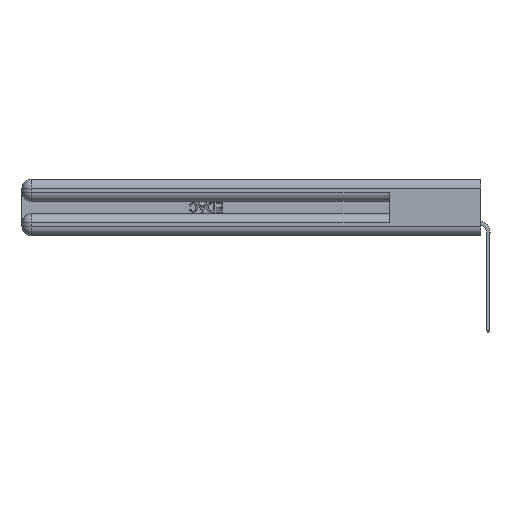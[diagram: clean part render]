
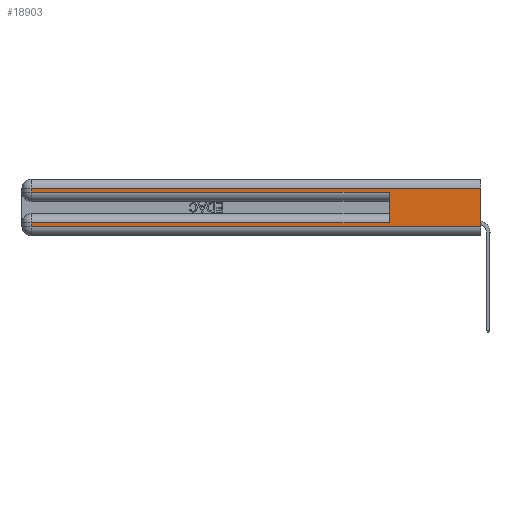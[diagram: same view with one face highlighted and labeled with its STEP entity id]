
A CAD part, left-side view. The second image highlights one B-rep face of the part: STEP entity #18903.
In plain terms, the highlighted planar face has unit normal (-1, 0, 0).
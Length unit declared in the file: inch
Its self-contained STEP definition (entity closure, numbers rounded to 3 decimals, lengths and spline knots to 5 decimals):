
#931 = ORIENTED_EDGE ( 'NONE', *, *, #13515, .T. ) ;
#1380 = EDGE_CURVE ( 'NONE', #7240, #13594, #26486, .T. ) ;
#1439 = VECTOR ( 'NONE', #4902, 39.37008 ) ;
#1714 = CARTESIAN_POINT ( 'NONE',  ( 0., 2.94, 0.31 ) ) ;
#1942 = VECTOR ( 'NONE', #2639, 39.37008 ) ;
#2200 = DIRECTION ( 'NONE',  ( 0., 0., -1. ) ) ;
#2639 = DIRECTION ( 'NONE',  ( 0., 0., 1. ) ) ;
#2645 = LINE ( 'NONE', #15497, #1439 ) ;
#2689 = VERTEX_POINT ( 'NONE', #3376 ) ;
#3376 = CARTESIAN_POINT ( 'NONE',  ( 0., 0., 0.31 ) ) ;
#4289 = CARTESIAN_POINT ( 'NONE',  ( 0., 0., 0.37 ) ) ;
#4371 = EDGE_CURVE ( 'NONE', #7240, #5179, #33213, .T. ) ;
#4902 = DIRECTION ( 'NONE',  ( 0., -1., 0. ) ) ;
#5179 = VERTEX_POINT ( 'NONE', #25873 ) ;
#5207 = EDGE_CURVE ( 'NONE', #2689, #12162, #29871, .T. ) ;
#6254 = CARTESIAN_POINT ( 'NONE',  ( 0., 0.6, 0.085 ) ) ;
#7240 = VERTEX_POINT ( 'NONE', #6254 ) ;
#7918 = LINE ( 'NONE', #9277, #29573 ) ;
#8537 = ORIENTED_EDGE ( 'NONE', *, *, #27252, .F. ) ;
#9277 = CARTESIAN_POINT ( 'NONE',  ( 0., 2.94, 0.37 ) ) ;
#9321 = CARTESIAN_POINT ( 'NONE',  ( 0., 0., 0.06 ) ) ;
#10846 = VERTEX_POINT ( 'NONE', #32232 ) ;
#11100 = CARTESIAN_POINT ( 'NONE',  ( 0., 0.6, 0.285 ) ) ;
#11950 = VERTEX_POINT ( 'NONE', #21241 ) ;
#12162 = VERTEX_POINT ( 'NONE', #1714 ) ;
#12585 = FACE_OUTER_BOUND ( 'NONE', #28027, .T. ) ;
#12938 = CARTESIAN_POINT ( 'NONE',  ( 0., 0., 0.06 ) ) ;
#13391 = VECTOR ( 'NONE', #2200, 39.37008 ) ;
#13396 = DIRECTION ( 'NONE',  ( 0., 1., 0. ) ) ;
#13515 = EDGE_CURVE ( 'NONE', #12162, #11950, #13818, .T. ) ;
#13594 = VERTEX_POINT ( 'NONE', #11100 ) ;
#13818 = LINE ( 'NONE', #28677, #13391 ) ;
#14566 = PLANE ( 'NONE',  #22147 ) ;
#14887 = ORIENTED_EDGE ( 'NONE', *, *, #5207, .T. ) ;
#15438 = DIRECTION ( 'NONE',  ( 0., -1., 0. ) ) ;
#15471 = EDGE_CURVE ( 'NONE', #11950, #13594, #2645, .T. ) ;
#15497 = CARTESIAN_POINT ( 'NONE',  ( 0., 0., 0.285 ) ) ;
#15861 = ORIENTED_EDGE ( 'NONE', *, *, #32471, .T. ) ;
#17479 = DIRECTION ( 'NONE',  ( 0., 0., -1. ) ) ;
#17927 = DIRECTION ( 'NONE',  ( 0., 1., 0. ) ) ;
#18652 = CARTESIAN_POINT ( 'NONE',  ( 0., 0., 0.31 ) ) ;
#18903 = ADVANCED_FACE ( 'NONE', ( #12585 ), #14566, .F. ) ;
#19794 = ORIENTED_EDGE ( 'NONE', *, *, #15471, .T. ) ;
#20044 = DIRECTION ( 'NONE',  ( 1., 0., 0. ) ) ;
#20277 = VECTOR ( 'NONE', #24504, 39.37008 ) ;
#21241 = CARTESIAN_POINT ( 'NONE',  ( 0., 2.94, 0.285 ) ) ;
#21288 = VECTOR ( 'NONE', #13396, 39.37008 ) ;
#21293 = LINE ( 'NONE', #12938, #31121 ) ;
#22147 = AXIS2_PLACEMENT_3D ( 'NONE', #4289, #20044, #32945 ) ;
#22194 = CARTESIAN_POINT ( 'NONE',  ( 0., 0., 0.085 ) ) ;
#22264 = ORIENTED_EDGE ( 'NONE', *, *, #33734, .T. ) ;
#24391 = LINE ( 'NONE', #27129, #20277 ) ;
#24504 = DIRECTION ( 'NONE',  ( 0., 0., -1. ) ) ;
#24622 = VERTEX_POINT ( 'NONE', #9321 ) ;
#25480 = VECTOR ( 'NONE', #17927, 39.37008 ) ;
#25656 = ORIENTED_EDGE ( 'NONE', *, *, #1380, .F. ) ;
#25873 = CARTESIAN_POINT ( 'NONE',  ( 0., 2.94, 0.085 ) ) ;
#26486 = LINE ( 'NONE', #33362, #1942 ) ;
#27129 = CARTESIAN_POINT ( 'NONE',  ( 0., 0., 0.37 ) ) ;
#27252 = EDGE_CURVE ( 'NONE', #2689, #24622, #24391, .T. ) ;
#28027 = EDGE_LOOP ( 'NONE', ( #8537, #14887, #931, #19794, #25656, #29530, #15861, #22264 ) ) ;
#28677 = CARTESIAN_POINT ( 'NONE',  ( 0., 2.94, 0.37 ) ) ;
#29530 = ORIENTED_EDGE ( 'NONE', *, *, #4371, .T. ) ;
#29573 = VECTOR ( 'NONE', #17479, 39.37008 ) ;
#29871 = LINE ( 'NONE', #18652, #21288 ) ;
#31121 = VECTOR ( 'NONE', #15438, 39.37008 ) ;
#32232 = CARTESIAN_POINT ( 'NONE',  ( 0., 2.94, 0.06 ) ) ;
#32471 = EDGE_CURVE ( 'NONE', #5179, #10846, #7918, .T. ) ;
#32945 = DIRECTION ( 'NONE',  ( 0., 0., -1. ) ) ;
#33213 = LINE ( 'NONE', #22194, #25480 ) ;
#33362 = CARTESIAN_POINT ( 'NONE',  ( 0., 0.6, 0.145 ) ) ;
#33734 = EDGE_CURVE ( 'NONE', #10846, #24622, #21293, .T. ) ;
